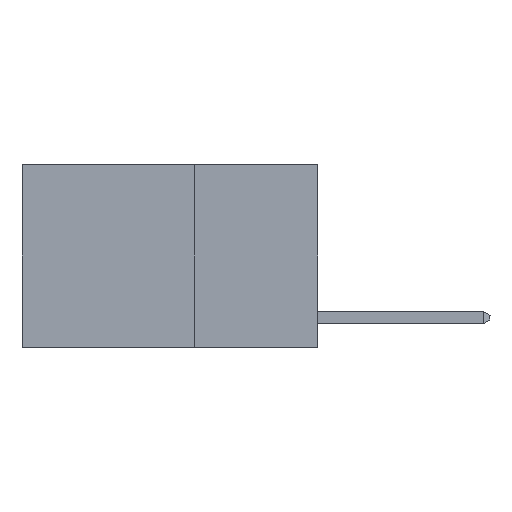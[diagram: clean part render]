
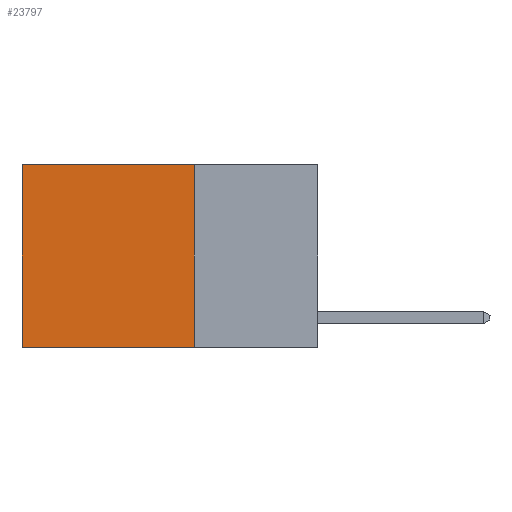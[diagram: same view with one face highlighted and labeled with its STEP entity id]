
A CAD part, left-side view. The second image highlights one B-rep face of the part: STEP entity #23797.
In plain terms, the highlighted planar face has unit normal (-1, 0, 0).
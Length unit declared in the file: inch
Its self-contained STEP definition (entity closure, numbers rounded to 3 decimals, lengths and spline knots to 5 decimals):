
#404 = ORIENTED_EDGE ( 'NONE', *, *, #8224, .T. ) ;
#1266 = EDGE_CURVE ( 'NONE', #4338, #19184, #15119, .T. ) ;
#2214 = LINE ( 'NONE', #15094, #18228 ) ;
#2813 = LINE ( 'NONE', #12454, #20650 ) ;
#2852 = VECTOR ( 'NONE', #8018, 39.37008 ) ;
#3593 = VERTEX_POINT ( 'NONE', #4965 ) ;
#4338 = VERTEX_POINT ( 'NONE', #11512 ) ;
#4357 = ORIENTED_EDGE ( 'NONE', *, *, #21569, .T. ) ;
#4965 = CARTESIAN_POINT ( 'NONE',  ( 0.2625, 0.6, 0. ) ) ;
#6943 = VERTEX_POINT ( 'NONE', #8765 ) ;
#7933 = CARTESIAN_POINT ( 'NONE',  ( 0.2625, 0.6, 0. ) ) ;
#8018 = DIRECTION ( 'NONE',  ( 0., 0., -1. ) ) ;
#8224 = EDGE_CURVE ( 'NONE', #4338, #3593, #2813, .T. ) ;
#8765 = CARTESIAN_POINT ( 'NONE',  ( 0.2625, 0.6, -0.37 ) ) ;
#10084 = CARTESIAN_POINT ( 'NONE',  ( 0.2625, 0.25, 0. ) ) ;
#11145 = PLANE ( 'NONE',  #18117 ) ;
#11512 = CARTESIAN_POINT ( 'NONE',  ( 0.2625, 0.25, 0. ) ) ;
#12454 = CARTESIAN_POINT ( 'NONE',  ( 0.2625, 0.25, 0. ) ) ;
#13056 = CARTESIAN_POINT ( 'NONE',  ( 0.2625, 0.25, 0. ) ) ;
#13119 = FACE_OUTER_BOUND ( 'NONE', #17144, .T. ) ;
#14426 = DIRECTION ( 'NONE',  ( 0., 1., 0. ) ) ;
#15094 = CARTESIAN_POINT ( 'NONE',  ( 0.2625, 0.25, -0.37 ) ) ;
#15119 = LINE ( 'NONE', #10084, #17202 ) ;
#15573 = ORIENTED_EDGE ( 'NONE', *, *, #22397, .F. ) ;
#15780 = ORIENTED_EDGE ( 'NONE', *, *, #1266, .F. ) ;
#16870 = DIRECTION ( 'NONE',  ( 1., 0., 0. ) ) ;
#17083 = LINE ( 'NONE', #7933, #2852 ) ;
#17144 = EDGE_LOOP ( 'NONE', ( #4357, #15573, #15780, #404 ) ) ;
#17202 = VECTOR ( 'NONE', #19532, 39.37008 ) ;
#18117 = AXIS2_PLACEMENT_3D ( 'NONE', #13056, #16870, #18840 ) ;
#18228 = VECTOR ( 'NONE', #18562, 39.37008 ) ;
#18562 = DIRECTION ( 'NONE',  ( 0., 1., 0. ) ) ;
#18840 = DIRECTION ( 'NONE',  ( 0., 0., -1. ) ) ;
#19184 = VERTEX_POINT ( 'NONE', #20170 ) ;
#19532 = DIRECTION ( 'NONE',  ( 0., 0., -1. ) ) ;
#20170 = CARTESIAN_POINT ( 'NONE',  ( 0.2625, 0.25, -0.37 ) ) ;
#20650 = VECTOR ( 'NONE', #14426, 39.37008 ) ;
#21569 = EDGE_CURVE ( 'NONE', #3593, #6943, #17083, .T. ) ;
#22397 = EDGE_CURVE ( 'NONE', #19184, #6943, #2214, .T. ) ;
#23797 = ADVANCED_FACE ( 'NONE', ( #13119 ), #11145, .F. ) ;
